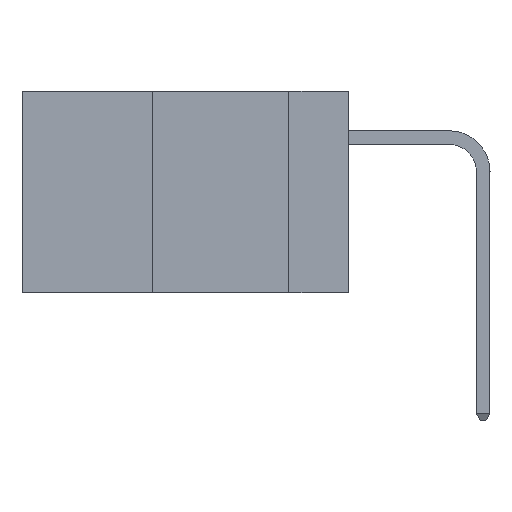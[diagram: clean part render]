
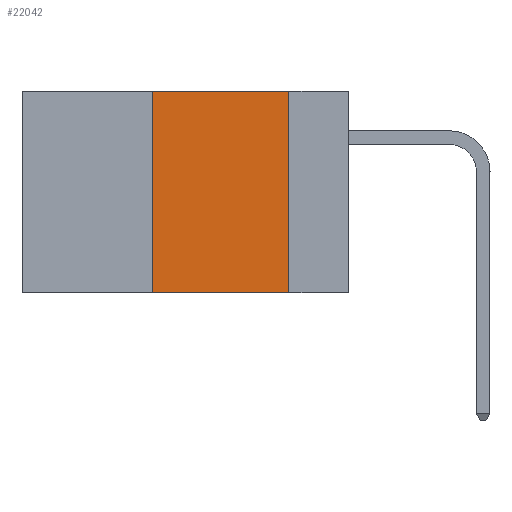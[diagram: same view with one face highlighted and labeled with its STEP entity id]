
A CAD part, left-side view. The second image highlights one B-rep face of the part: STEP entity #22042.
In plain terms, the highlighted planar face has unit normal (-1, 0, 0).
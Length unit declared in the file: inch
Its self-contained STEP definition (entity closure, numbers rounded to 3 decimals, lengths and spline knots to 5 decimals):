
#345 = DIRECTION ( 'NONE',  ( 0., -1., 0. ) ) ;
#1808 = VECTOR ( 'NONE', #18931, 39.37008 ) ;
#3909 = CARTESIAN_POINT ( 'NONE',  ( 0., 0.6, 0. ) ) ;
#4115 = EDGE_CURVE ( 'NONE', #11128, #7110, #4784, .T. ) ;
#4784 = LINE ( 'NONE', #3909, #8409 ) ;
#5318 = ORIENTED_EDGE ( 'NONE', *, *, #5593, .F. ) ;
#5593 = EDGE_CURVE ( 'NONE', #6990, #11128, #19324, .T. ) ;
#5886 = CARTESIAN_POINT ( 'NONE',  ( 0., 0.36, 0. ) ) ;
#6050 = EDGE_CURVE ( 'NONE', #6990, #21649, #13999, .T. ) ;
#6990 = VERTEX_POINT ( 'NONE', #12153 ) ;
#7110 = VERTEX_POINT ( 'NONE', #11284 ) ;
#7420 = CARTESIAN_POINT ( 'NONE',  ( 0., 0.6, -0.37 ) ) ;
#8381 = ORIENTED_EDGE ( 'NONE', *, *, #21638, .F. ) ;
#8409 = VECTOR ( 'NONE', #16475, 39.37008 ) ;
#8774 = DIRECTION ( 'NONE',  ( 1., 0., 0. ) ) ;
#8835 = EDGE_LOOP ( 'NONE', ( #8381, #18528, #5318, #20237 ) ) ;
#9463 = AXIS2_PLACEMENT_3D ( 'NONE', #19549, #8774, #21344 ) ;
#11128 = VERTEX_POINT ( 'NONE', #5886 ) ;
#11284 = CARTESIAN_POINT ( 'NONE',  ( 0., 0.11, 0. ) ) ;
#11927 = LINE ( 'NONE', #13541, #1808 ) ;
#12153 = CARTESIAN_POINT ( 'NONE',  ( 0., 0.36, -0.37 ) ) ;
#12368 = PLANE ( 'NONE',  #9463 ) ;
#13541 = CARTESIAN_POINT ( 'NONE',  ( 0., 0.11, 0. ) ) ;
#13999 = LINE ( 'NONE', #7420, #18165 ) ;
#15174 = DIRECTION ( 'NONE',  ( 0., 0., 1. ) ) ;
#15408 = CARTESIAN_POINT ( 'NONE',  ( 0., 0.11, -0.37 ) ) ;
#16081 = FACE_OUTER_BOUND ( 'NONE', #8835, .T. ) ;
#16475 = DIRECTION ( 'NONE',  ( 0., -1., 0. ) ) ;
#18165 = VECTOR ( 'NONE', #345, 39.37008 ) ;
#18528 = ORIENTED_EDGE ( 'NONE', *, *, #4115, .F. ) ;
#18772 = CARTESIAN_POINT ( 'NONE',  ( 0., 0.36, 0. ) ) ;
#18931 = DIRECTION ( 'NONE',  ( 0., 0., -1. ) ) ;
#19324 = LINE ( 'NONE', #18772, #22913 ) ;
#19549 = CARTESIAN_POINT ( 'NONE',  ( 0., 0.6, 0. ) ) ;
#20237 = ORIENTED_EDGE ( 'NONE', *, *, #6050, .T. ) ;
#21344 = DIRECTION ( 'NONE',  ( 0., 0., -1. ) ) ;
#21638 = EDGE_CURVE ( 'NONE', #7110, #21649, #11927, .T. ) ;
#21649 = VERTEX_POINT ( 'NONE', #15408 ) ;
#22042 = ADVANCED_FACE ( 'NONE', ( #16081 ), #12368, .F. ) ;
#22913 = VECTOR ( 'NONE', #15174, 39.37008 ) ;
